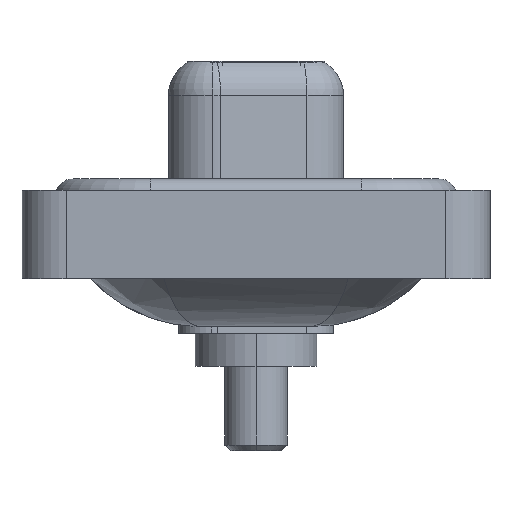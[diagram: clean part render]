
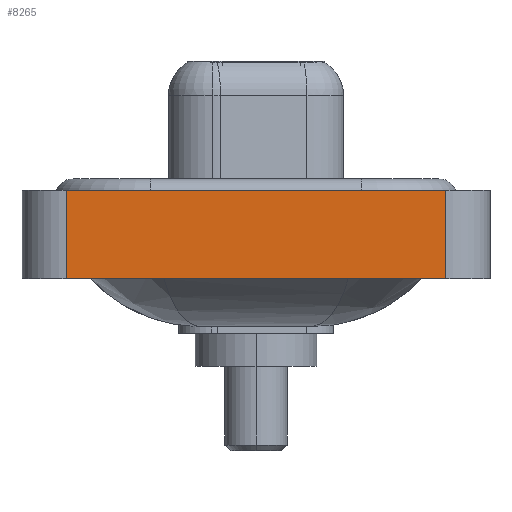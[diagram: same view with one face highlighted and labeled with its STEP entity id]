
A CAD part, left-side view. The second image highlights one B-rep face of the part: STEP entity #8265.
In plain terms, the highlighted planar face has unit normal (-1, 0, 0).
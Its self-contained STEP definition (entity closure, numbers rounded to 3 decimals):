
#183 = DIRECTION ( 'NONE',  ( 0., 0., 1. ) ) ;
#617 = CARTESIAN_POINT ( 'NONE',  ( -7.25, 8.55, -3.6 ) ) ;
#785 = FACE_OUTER_BOUND ( 'NONE', #4055, .T. ) ;
#1243 = VERTEX_POINT ( 'NONE', #16470 ) ;
#2084 = CARTESIAN_POINT ( 'NONE',  ( -7.25, -8.55, 0.4 ) ) ;
#2105 = ORIENTED_EDGE ( 'NONE', *, *, #7554, .T. ) ;
#2962 = EDGE_CURVE ( 'NONE', #11096, #1243, #9606, .T. ) ;
#3083 = ORIENTED_EDGE ( 'NONE', *, *, #15586, .F. ) ;
#3085 = VERTEX_POINT ( 'NONE', #15042 ) ;
#4055 = EDGE_LOOP ( 'NONE', ( #4505, #5484, #3083, #2105 ) ) ;
#4341 = VERTEX_POINT ( 'NONE', #7122 ) ;
#4505 = ORIENTED_EDGE ( 'NONE', *, *, #2962, .T. ) ;
#5484 = ORIENTED_EDGE ( 'NONE', *, *, #7733, .F. ) ;
#5814 = DIRECTION ( 'NONE',  ( 0., -1., 0. ) ) ;
#5951 = PLANE ( 'NONE',  #10813 ) ;
#6954 = LINE ( 'NONE', #617, #8313 ) ;
#7122 = CARTESIAN_POINT ( 'NONE',  ( -7.25, 8.55, -3.6 ) ) ;
#7166 = LINE ( 'NONE', #2084, #12912 ) ;
#7554 = EDGE_CURVE ( 'NONE', #4341, #11096, #13050, .T. ) ;
#7733 = EDGE_CURVE ( 'NONE', #3085, #1243, #7166, .T. ) ;
#8265 = ADVANCED_FACE ( 'NONE', ( #785 ), #5951, .T. ) ;
#8313 = VECTOR ( 'NONE', #16101, 1000. ) ;
#9073 = VECTOR ( 'NONE', #14717, 1000. ) ;
#9154 = DIRECTION ( 'NONE',  ( -1., 0., 0. ) ) ;
#9606 = LINE ( 'NONE', #13212, #9073 ) ;
#9695 = CARTESIAN_POINT ( 'NONE',  ( -7.25, -8.55, -3.6 ) ) ;
#10813 = AXIS2_PLACEMENT_3D ( 'NONE', #15424, #9154, #183 ) ;
#11096 = VERTEX_POINT ( 'NONE', #9695 ) ;
#12912 = VECTOR ( 'NONE', #5814, 1000. ) ;
#13050 = LINE ( 'NONE', #14323, #16110 ) ;
#13212 = CARTESIAN_POINT ( 'NONE',  ( -7.25, -8.55, -3.6 ) ) ;
#14323 = CARTESIAN_POINT ( 'NONE',  ( -7.25, -8.55, -3.6 ) ) ;
#14484 = DIRECTION ( 'NONE',  ( 0., -1., 0. ) ) ;
#14717 = DIRECTION ( 'NONE',  ( 0., 0., 1. ) ) ;
#15042 = CARTESIAN_POINT ( 'NONE',  ( -7.25, 8.55, 0.4 ) ) ;
#15424 = CARTESIAN_POINT ( 'NONE',  ( -7.25, -8.55, -3.6 ) ) ;
#15586 = EDGE_CURVE ( 'NONE', #4341, #3085, #6954, .T. ) ;
#16101 = DIRECTION ( 'NONE',  ( 0., 0., 1. ) ) ;
#16110 = VECTOR ( 'NONE', #14484, 1000. ) ;
#16470 = CARTESIAN_POINT ( 'NONE',  ( -7.25, -8.55, 0.4 ) ) ;
